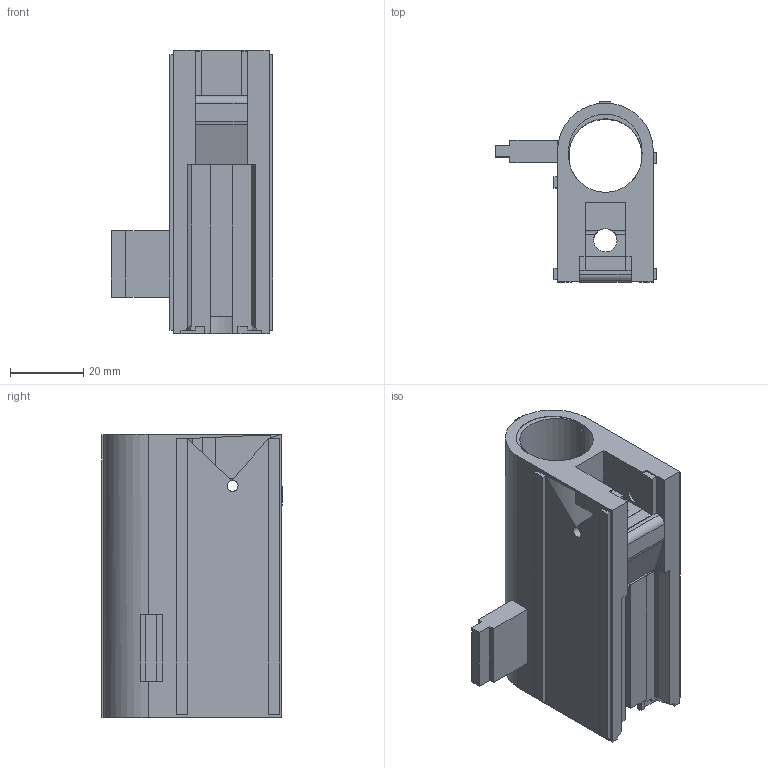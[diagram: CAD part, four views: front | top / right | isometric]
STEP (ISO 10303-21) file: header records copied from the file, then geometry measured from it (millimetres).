
FILE_DESCRIPTION (( 'STEP AP203' ), '1' );
FILE_NAME ('WTF-9_updated_bolt_housing.STEP', '2020-06-16T21:39:27', ( '' ), ( '' ), 'SwSTEP 2.0', 'SolidWorks 2016', '' );
FILE_SCHEMA (( 'CONFIG_CONTROL_DESIGN' ));
Length unit declared in the file: millimetre
Products named in the file (1): WTF-9_updated_bolt_housing
Bounding box: 44 x 49.1 x 77.19 mm (x, y, z)
Volume: 45389.6 mm3; surface area: 22424.1 mm2
Topology: 3 solids, 3 shells, 161 faces, 450 edges, 299 vertices
Faces by surface type: plane 144, cylinder 17
Full cylindrical faces by diameter (mm): 2.968 x2, 3 x1, 3.566 x1, 6.34 x1, 20 x1
Entity records: 5282 total; most frequent: CARTESIAN_POINT 1061, ORIENTED_EDGE 884, DIRECTION 803, EDGE_CURVE 442, VECTOR 381, LINE 381, VERTEX_POINT 297, AXIS2_PLACEMENT_3D 211
